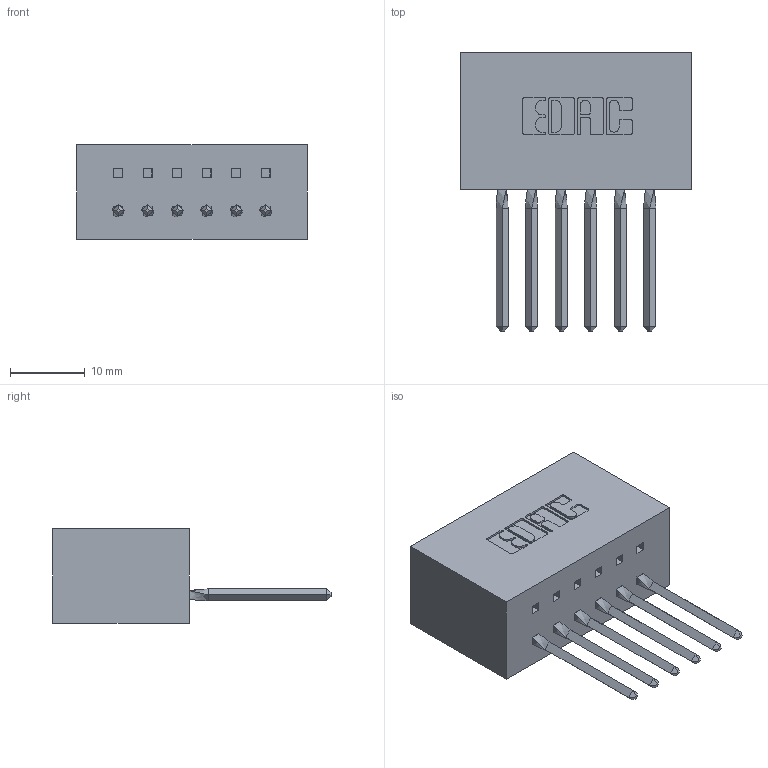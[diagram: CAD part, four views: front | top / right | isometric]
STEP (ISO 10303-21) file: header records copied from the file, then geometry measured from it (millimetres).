
FILE_DESCRIPTION (( 'STEP AP203' ), '1' );
FILE_NAME ('317-006-541-601.STEP', '2020-02-27T12:43:14', ( '' ), ( '' ), 'SwSTEP 2.0', 'SolidWorks 2016', '' );
FILE_SCHEMA (( 'CONFIG_CONTROL_DESIGN' ));
Length unit declared in the file: inch
Products named in the file (3): 317-006-541-601; 317-290-002_541; 317 Part_Lugless
Assembly tree (7 placements, depth 2):
  317-006-541-601
    317 Part_Lugless
    317-290-002_541  x6
Bounding box: 30.99 x 37.34 x 12.7 mm (x, y, z)
Volume: 5624.1 mm3; surface area: 6940.7 mm2
Topology: 7 solids, 7 shells, 1002 faces, 2843 edges, 1850 vertices
Faces by surface type: plane 794, cylinder 184, bspline 24
Entity records: 14642 total; most frequent: CARTESIAN_POINT 3227, ORIENTED_EDGE 2486, DIRECTION 2007, EDGE_CURVE 1243, LINE 887, VECTOR 887, VERTEX_POINT 820, AXIS2_PLACEMENT_3D 560
